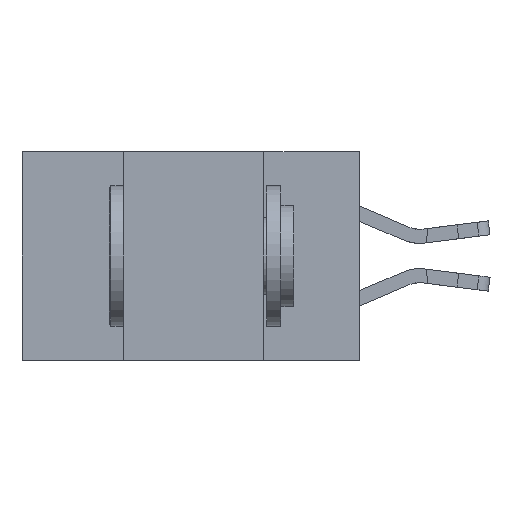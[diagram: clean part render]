
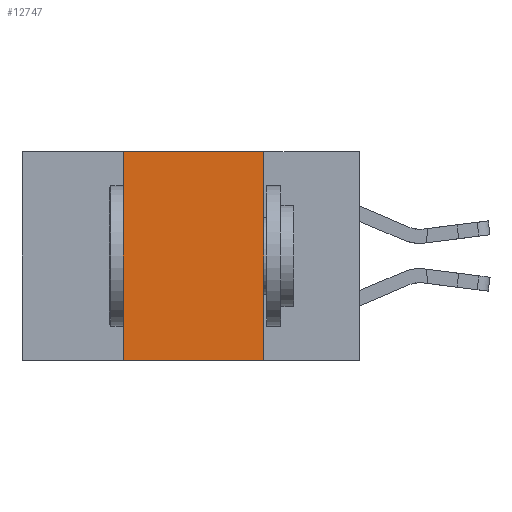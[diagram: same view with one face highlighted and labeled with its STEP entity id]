
A CAD part, left-side view. The second image highlights one B-rep face of the part: STEP entity #12747.
In plain terms, the highlighted planar face has unit normal (-1, 0, 0).
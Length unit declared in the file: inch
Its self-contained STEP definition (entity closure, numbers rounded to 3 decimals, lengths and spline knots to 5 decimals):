
#1328 = CARTESIAN_POINT ( 'NONE',  ( 0., 0.42, 0. ) ) ;
#1365 = CARTESIAN_POINT ( 'NONE',  ( 0., 0.42, 0. ) ) ;
#2018 = LINE ( 'NONE', #13695, #6050 ) ;
#2156 = ORIENTED_EDGE ( 'NONE', *, *, #13709, .F. ) ;
#3734 = ORIENTED_EDGE ( 'NONE', *, *, #28737, .F. ) ;
#3928 = VECTOR ( 'NONE', #24185, 39.37008 ) ;
#3968 = EDGE_CURVE ( 'NONE', #17062, #24981, #16071, .T. ) ;
#4000 = EDGE_CURVE ( 'NONE', #29451, #12807, #21275, .T. ) ;
#4703 = VECTOR ( 'NONE', #26349, 39.37008 ) ;
#6050 = VECTOR ( 'NONE', #20415, 39.37008 ) ;
#11532 = EDGE_LOOP ( 'NONE', ( #2156, #22907, #3734, #16311 ) ) ;
#12747 = ADVANCED_FACE ( 'NONE', ( #20895 ), #12761, .F. ) ;
#12761 = PLANE ( 'NONE',  #20986 ) ;
#12768 = CARTESIAN_POINT ( 'NONE',  ( 0., 0.6, 0. ) ) ;
#12807 = VERTEX_POINT ( 'NONE', #28735 ) ;
#13458 = CARTESIAN_POINT ( 'NONE',  ( 0., 0.17, -0.37 ) ) ;
#13695 = CARTESIAN_POINT ( 'NONE',  ( 0., 0.17, 0. ) ) ;
#13709 = EDGE_CURVE ( 'NONE', #12807, #24981, #2018, .T. ) ;
#15000 = DIRECTION ( 'NONE',  ( 0., 0., -1. ) ) ;
#15209 = DIRECTION ( 'NONE',  ( 0., -1., 0. ) ) ;
#15345 = VECTOR ( 'NONE', #15209, 39.37008 ) ;
#16071 = LINE ( 'NONE', #21853, #3928 ) ;
#16311 = ORIENTED_EDGE ( 'NONE', *, *, #3968, .T. ) ;
#17062 = VERTEX_POINT ( 'NONE', #20179 ) ;
#20179 = CARTESIAN_POINT ( 'NONE',  ( 0., 0.42, -0.37 ) ) ;
#20415 = DIRECTION ( 'NONE',  ( 0., 0., -1. ) ) ;
#20895 = FACE_OUTER_BOUND ( 'NONE', #11532, .T. ) ;
#20986 = AXIS2_PLACEMENT_3D ( 'NONE', #23980, #28545, #15000 ) ;
#21275 = LINE ( 'NONE', #12768, #15345 ) ;
#21853 = CARTESIAN_POINT ( 'NONE',  ( 0., 0.6, -0.37 ) ) ;
#22750 = LINE ( 'NONE', #1365, #4703 ) ;
#22907 = ORIENTED_EDGE ( 'NONE', *, *, #4000, .F. ) ;
#23980 = CARTESIAN_POINT ( 'NONE',  ( 0., 0.6, 0. ) ) ;
#24185 = DIRECTION ( 'NONE',  ( 0., -1., 0. ) ) ;
#24981 = VERTEX_POINT ( 'NONE', #13458 ) ;
#26349 = DIRECTION ( 'NONE',  ( 0., 0., 1. ) ) ;
#28545 = DIRECTION ( 'NONE',  ( 1., 0., 0. ) ) ;
#28735 = CARTESIAN_POINT ( 'NONE',  ( 0., 0.17, 0. ) ) ;
#28737 = EDGE_CURVE ( 'NONE', #17062, #29451, #22750, .T. ) ;
#29451 = VERTEX_POINT ( 'NONE', #1328 ) ;
